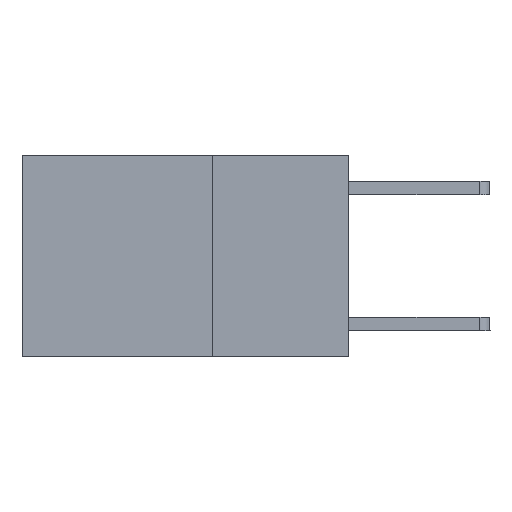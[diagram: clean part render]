
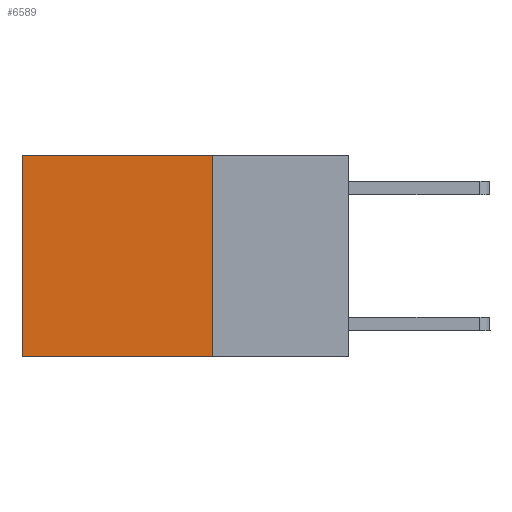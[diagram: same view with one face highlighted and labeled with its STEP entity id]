
A CAD part, left-side view. The second image highlights one B-rep face of the part: STEP entity #6589.
In plain terms, the highlighted planar face has unit normal (-1, 0, 0).
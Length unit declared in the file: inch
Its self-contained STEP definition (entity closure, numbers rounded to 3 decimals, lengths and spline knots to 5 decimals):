
#167 = VERTEX_POINT ( 'NONE', #844 ) ;
#247 = DIRECTION ( 'NONE',  ( 0., 1., 0. ) ) ;
#844 = CARTESIAN_POINT ( 'NONE',  ( 0.2625, 0.25, 0. ) ) ;
#967 = CARTESIAN_POINT ( 'NONE',  ( 0.2625, 0.6, 0. ) ) ;
#1095 = DIRECTION ( 'NONE',  ( 0., 0., -1. ) ) ;
#1214 = DIRECTION ( 'NONE',  ( 0., 1., 0. ) ) ;
#1803 = LINE ( 'NONE', #9546, #3315 ) ;
#2655 = EDGE_CURVE ( 'NONE', #167, #3266, #7110, .T. ) ;
#2681 = PLANE ( 'NONE',  #3880 ) ;
#2974 = EDGE_CURVE ( 'NONE', #3266, #6185, #1803, .T. ) ;
#3266 = VERTEX_POINT ( 'NONE', #967 ) ;
#3315 = VECTOR ( 'NONE', #5922, 39.37008 ) ;
#3504 = ORIENTED_EDGE ( 'NONE', *, *, #2655, .T. ) ;
#3536 = ORIENTED_EDGE ( 'NONE', *, *, #6561, .F. ) ;
#3880 = AXIS2_PLACEMENT_3D ( 'NONE', #7815, #5529, #1095 ) ;
#3919 = ORIENTED_EDGE ( 'NONE', *, *, #2974, .T. ) ;
#4035 = ORIENTED_EDGE ( 'NONE', *, *, #4810, .F. ) ;
#4083 = CARTESIAN_POINT ( 'NONE',  ( 0.2625, 0.25, -0.37 ) ) ;
#4247 = CARTESIAN_POINT ( 'NONE',  ( 0.2625, 0.25, 0. ) ) ;
#4810 = EDGE_CURVE ( 'NONE', #7185, #6185, #9565, .T. ) ;
#5145 = VECTOR ( 'NONE', #1214, 39.37008 ) ;
#5467 = CARTESIAN_POINT ( 'NONE',  ( 0.2625, 0.25, 0. ) ) ;
#5529 = DIRECTION ( 'NONE',  ( 1., 0., 0. ) ) ;
#5922 = DIRECTION ( 'NONE',  ( 0., 0., -1. ) ) ;
#6185 = VERTEX_POINT ( 'NONE', #9334 ) ;
#6561 = EDGE_CURVE ( 'NONE', #167, #7185, #8663, .T. ) ;
#6589 = ADVANCED_FACE ( 'NONE', ( #8873 ), #2681, .F. ) ;
#6606 = VECTOR ( 'NONE', #7778, 39.37008 ) ;
#7110 = LINE ( 'NONE', #4247, #5145 ) ;
#7185 = VERTEX_POINT ( 'NONE', #8560 ) ;
#7265 = VECTOR ( 'NONE', #247, 39.37008 ) ;
#7778 = DIRECTION ( 'NONE',  ( 0., 0., -1. ) ) ;
#7815 = CARTESIAN_POINT ( 'NONE',  ( 0.2625, 0.25, 0. ) ) ;
#7959 = EDGE_LOOP ( 'NONE', ( #3919, #4035, #3536, #3504 ) ) ;
#8560 = CARTESIAN_POINT ( 'NONE',  ( 0.2625, 0.25, -0.37 ) ) ;
#8663 = LINE ( 'NONE', #5467, #6606 ) ;
#8873 = FACE_OUTER_BOUND ( 'NONE', #7959, .T. ) ;
#9334 = CARTESIAN_POINT ( 'NONE',  ( 0.2625, 0.6, -0.37 ) ) ;
#9546 = CARTESIAN_POINT ( 'NONE',  ( 0.2625, 0.6, 0. ) ) ;
#9565 = LINE ( 'NONE', #4083, #7265 ) ;
